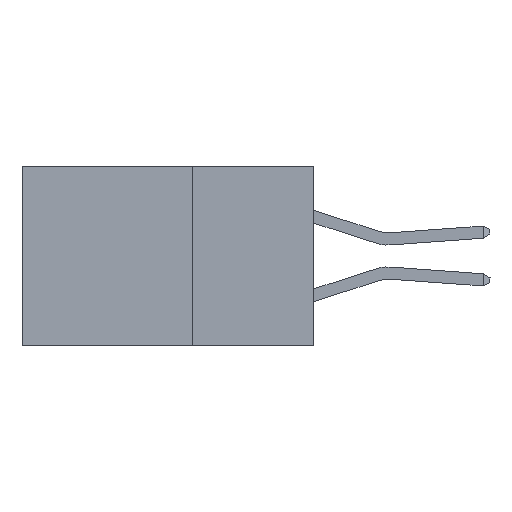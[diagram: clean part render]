
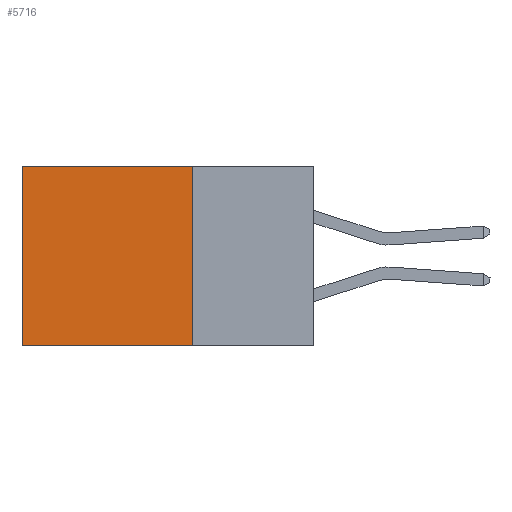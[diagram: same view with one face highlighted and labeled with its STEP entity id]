
A CAD part, left-side view. The second image highlights one B-rep face of the part: STEP entity #5716.
In plain terms, the highlighted planar face has unit normal (-1, 0, 0).
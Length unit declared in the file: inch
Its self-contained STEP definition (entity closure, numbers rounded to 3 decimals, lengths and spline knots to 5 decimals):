
#206 = AXIS2_PLACEMENT_3D ( 'NONE', #5337, #1995, #7823 ) ;
#334 = LINE ( 'NONE', #3607, #2448 ) ;
#371 = EDGE_CURVE ( 'NONE', #5264, #8337, #8903, .T. ) ;
#644 = VECTOR ( 'NONE', #8065, 39.37008 ) ;
#1880 = EDGE_CURVE ( 'NONE', #9297, #5264, #3255, .T. ) ;
#1995 = DIRECTION ( 'NONE',  ( 1., 0., 0. ) ) ;
#2448 = VECTOR ( 'NONE', #8533, 39.37008 ) ;
#2457 = DIRECTION ( 'NONE',  ( 0., 1., 0. ) ) ;
#2720 = CARTESIAN_POINT ( 'NONE',  ( 0.2875, 0.6, -0.37 ) ) ;
#2992 = LINE ( 'NONE', #4999, #9283 ) ;
#3162 = CARTESIAN_POINT ( 'NONE',  ( 0.2875, 0.6, 0. ) ) ;
#3255 = LINE ( 'NONE', #7366, #644 ) ;
#3607 = CARTESIAN_POINT ( 'NONE',  ( 0.2875, 0.25, 0. ) ) ;
#3892 = CARTESIAN_POINT ( 'NONE',  ( 0.2875, 0.6, 0. ) ) ;
#4401 = ORIENTED_EDGE ( 'NONE', *, *, #9649, .F. ) ;
#4574 = VECTOR ( 'NONE', #10828, 39.37008 ) ;
#4742 = FACE_OUTER_BOUND ( 'NONE', #6263, .T. ) ;
#4999 = CARTESIAN_POINT ( 'NONE',  ( 0.2875, 0.25, -0.37 ) ) ;
#5083 = VERTEX_POINT ( 'NONE', #6091 ) ;
#5264 = VERTEX_POINT ( 'NONE', #3892 ) ;
#5337 = CARTESIAN_POINT ( 'NONE',  ( 0.2875, 0.25, 0. ) ) ;
#5716 = ADVANCED_FACE ( 'NONE', ( #4742 ), #6943, .F. ) ;
#6091 = CARTESIAN_POINT ( 'NONE',  ( 0.2875, 0.25, -0.37 ) ) ;
#6263 = EDGE_LOOP ( 'NONE', ( #10333, #8502, #4401, #8751 ) ) ;
#6449 = CARTESIAN_POINT ( 'NONE',  ( 0.2875, 0.25, 0. ) ) ;
#6943 = PLANE ( 'NONE',  #206 ) ;
#7042 = EDGE_CURVE ( 'NONE', #5083, #8337, #2992, .T. ) ;
#7366 = CARTESIAN_POINT ( 'NONE',  ( 0.2875, 0.25, 0. ) ) ;
#7823 = DIRECTION ( 'NONE',  ( 0., 0., -1. ) ) ;
#8065 = DIRECTION ( 'NONE',  ( 0., 1., 0. ) ) ;
#8337 = VERTEX_POINT ( 'NONE', #2720 ) ;
#8502 = ORIENTED_EDGE ( 'NONE', *, *, #7042, .F. ) ;
#8533 = DIRECTION ( 'NONE',  ( 0., 0., -1. ) ) ;
#8751 = ORIENTED_EDGE ( 'NONE', *, *, #1880, .T. ) ;
#8903 = LINE ( 'NONE', #3162, #4574 ) ;
#9283 = VECTOR ( 'NONE', #2457, 39.37008 ) ;
#9297 = VERTEX_POINT ( 'NONE', #6449 ) ;
#9649 = EDGE_CURVE ( 'NONE', #9297, #5083, #334, .T. ) ;
#10333 = ORIENTED_EDGE ( 'NONE', *, *, #371, .T. ) ;
#10828 = DIRECTION ( 'NONE',  ( 0., 0., -1. ) ) ;
